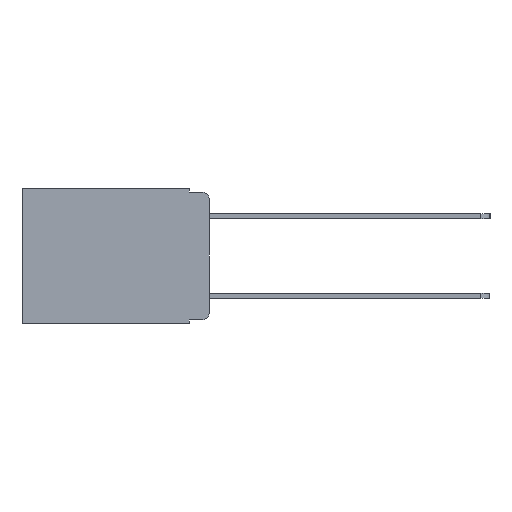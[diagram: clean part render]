
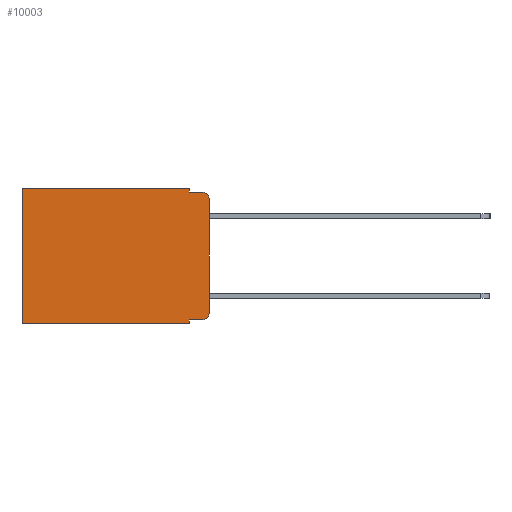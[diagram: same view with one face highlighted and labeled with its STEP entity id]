
A CAD part, left-side view. The second image highlights one B-rep face of the part: STEP entity #10003.
In plain terms, the highlighted planar face has unit normal (-1, 0, 0).
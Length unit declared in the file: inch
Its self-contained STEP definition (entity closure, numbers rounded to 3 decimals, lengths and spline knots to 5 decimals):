
#554 = ORIENTED_EDGE ( 'NONE', *, *, #4159, .T. ) ;
#816 = VERTEX_POINT ( 'NONE', #14394 ) ;
#1519 = VECTOR ( 'NONE', #15844, 39.37008 ) ;
#1655 = CARTESIAN_POINT ( 'NONE',  ( 0.298, 0.051, -0.01 ) ) ;
#2200 = DIRECTION ( 'NONE',  ( 0., 0., -1. ) ) ;
#2256 = EDGE_CURVE ( 'NONE', #7905, #13920, #16544, .T. ) ;
#2439 = LINE ( 'NONE', #9801, #15639 ) ;
#2563 = VERTEX_POINT ( 'NONE', #10602 ) ;
#3009 = CARTESIAN_POINT ( 'NONE',  ( 0.298, 0., -0.343 ) ) ;
#3080 = CARTESIAN_POINT ( 'NONE',  ( 0.298, 0.051, 0. ) ) ;
#3107 = ORIENTED_EDGE ( 'NONE', *, *, #4132, .F. ) ;
#3356 = ORIENTED_EDGE ( 'NONE', *, *, #2256, .T. ) ;
#3357 = CARTESIAN_POINT ( 'NONE',  ( 0.298, 0., -0.313 ) ) ;
#3617 = ORIENTED_EDGE ( 'NONE', *, *, #4163, .F. ) ;
#3933 = EDGE_CURVE ( 'NONE', #5489, #11102, #9654, .T. ) ;
#4132 = EDGE_CURVE ( 'NONE', #12912, #11701, #13716, .T. ) ;
#4159 = EDGE_CURVE ( 'NONE', #12912, #816, #13006, .T. ) ;
#4163 = EDGE_CURVE ( 'NONE', #6048, #816, #2439, .T. ) ;
#4187 = EDGE_CURVE ( 'NONE', #7905, #6048, #15972, .T. ) ;
#4191 = EDGE_CURVE ( 'NONE', #13920, #11102, #12296, .T. ) ;
#4195 = EDGE_CURVE ( 'NONE', #6336, #5489, #14955, .T. ) ;
#4214 = EDGE_CURVE ( 'NONE', #6336, #2563, #8811, .T. ) ;
#4217 = EDGE_CURVE ( 'NONE', #2563, #11701, #11612, .T. ) ;
#4826 = DIRECTION ( 'NONE',  ( 0., 0., -1. ) ) ;
#4884 = CARTESIAN_POINT ( 'NONE',  ( 0.298, 0.051, 0. ) ) ;
#4959 = ORIENTED_EDGE ( 'NONE', *, *, #4217, .T. ) ;
#5005 = VECTOR ( 'NONE', #4826, 39.37008 ) ;
#5280 = ORIENTED_EDGE ( 'NONE', *, *, #4214, .T. ) ;
#5489 = VERTEX_POINT ( 'NONE', #15394 ) ;
#5558 = DIRECTION ( 'NONE',  ( 0., 0., -1. ) ) ;
#5625 = CARTESIAN_POINT ( 'NONE',  ( 0.298, 0., 0. ) ) ;
#5723 = CARTESIAN_POINT ( 'NONE',  ( 0.298, 0., 0. ) ) ;
#5915 = CARTESIAN_POINT ( 'NONE',  ( 0.298, 0., -0.03 ) ) ;
#5949 = ORIENTED_EDGE ( 'NONE', *, *, #3933, .F. ) ;
#6048 = VERTEX_POINT ( 'NONE', #1655 ) ;
#6069 = DIRECTION ( 'NONE',  ( 0., -1., 0. ) ) ;
#6336 = VERTEX_POINT ( 'NONE', #8423 ) ;
#6429 = VECTOR ( 'NONE', #10568, 39.37008 ) ;
#7172 = VECTOR ( 'NONE', #12456, 39.37008 ) ;
#7332 = VECTOR ( 'NONE', #5558, 39.37008 ) ;
#7707 = DIRECTION ( 'NONE',  ( 0., 0., -1. ) ) ;
#7724 = DIRECTION ( 'NONE',  ( -1., 0., 0. ) ) ;
#7732 = CARTESIAN_POINT ( 'NONE',  ( 0.298, 0.02, -0.313 ) ) ;
#7905 = VERTEX_POINT ( 'NONE', #3080 ) ;
#8303 = AXIS2_PLACEMENT_3D ( 'NONE', #9540, #9524, #8873 ) ;
#8423 = CARTESIAN_POINT ( 'NONE',  ( 0.298, 0.051, -0.333 ) ) ;
#8775 = ORIENTED_EDGE ( 'NONE', *, *, #4187, .F. ) ;
#8811 = LINE ( 'NONE', #12923, #14241 ) ;
#8853 = DIRECTION ( 'NONE',  ( 0., -1., 0. ) ) ;
#8873 = DIRECTION ( 'NONE',  ( 0., 0., -1. ) ) ;
#9524 = DIRECTION ( 'NONE',  ( -1., 0., 0. ) ) ;
#9540 = CARTESIAN_POINT ( 'NONE',  ( 0.298, 0.02, -0.03 ) ) ;
#9553 = AXIS2_PLACEMENT_3D ( 'NONE', #5723, #16585, #9894 ) ;
#9654 = LINE ( 'NONE', #3009, #6429 ) ;
#9801 = CARTESIAN_POINT ( 'NONE',  ( 0.298, 0.051, -0.01 ) ) ;
#9894 = DIRECTION ( 'NONE',  ( 0., 0., -1. ) ) ;
#10003 = ADVANCED_FACE ( 'NONE', ( #15255 ), #12108, .F. ) ;
#10078 = EDGE_LOOP ( 'NONE', ( #3107, #554, #3617, #8775, #3356, #12429, #5949, #15469, #5280, #4959 ) ) ;
#10181 = CARTESIAN_POINT ( 'NONE',  ( 0.298, 0., 0. ) ) ;
#10568 = DIRECTION ( 'NONE',  ( 0., 1., 0. ) ) ;
#10602 = CARTESIAN_POINT ( 'NONE',  ( 0.298, 0.02, -0.333 ) ) ;
#11102 = VERTEX_POINT ( 'NONE', #15483 ) ;
#11612 = CIRCLE ( 'NONE', #12303, 0.02 ) ;
#11701 = VERTEX_POINT ( 'NONE', #3357 ) ;
#11951 = VECTOR ( 'NONE', #2200, 39.37008 ) ;
#12108 = PLANE ( 'NONE',  #9553 ) ;
#12296 = LINE ( 'NONE', #14493, #11951 ) ;
#12303 = AXIS2_PLACEMENT_3D ( 'NONE', #7732, #7724, #7707 ) ;
#12429 = ORIENTED_EDGE ( 'NONE', *, *, #4191, .T. ) ;
#12456 = DIRECTION ( 'NONE',  ( 0., 1., 0. ) ) ;
#12912 = VERTEX_POINT ( 'NONE', #5915 ) ;
#12923 = CARTESIAN_POINT ( 'NONE',  ( 0.298, 0.051, -0.333 ) ) ;
#13006 = CIRCLE ( 'NONE', #8303, 0.02 ) ;
#13716 = LINE ( 'NONE', #5625, #7332 ) ;
#13920 = VERTEX_POINT ( 'NONE', #16578 ) ;
#14241 = VECTOR ( 'NONE', #6069, 39.37008 ) ;
#14394 = CARTESIAN_POINT ( 'NONE',  ( 0.298, 0.02, -0.01 ) ) ;
#14493 = CARTESIAN_POINT ( 'NONE',  ( 0.298, 0.473, 0. ) ) ;
#14955 = LINE ( 'NONE', #4884, #5005 ) ;
#15255 = FACE_OUTER_BOUND ( 'NONE', #10078, .T. ) ;
#15394 = CARTESIAN_POINT ( 'NONE',  ( 0.298, 0.051, -0.343 ) ) ;
#15469 = ORIENTED_EDGE ( 'NONE', *, *, #4195, .F. ) ;
#15483 = CARTESIAN_POINT ( 'NONE',  ( 0.298, 0.473, -0.343 ) ) ;
#15639 = VECTOR ( 'NONE', #8853, 39.37008 ) ;
#15844 = DIRECTION ( 'NONE',  ( 0., 0., -1. ) ) ;
#15857 = CARTESIAN_POINT ( 'NONE',  ( 0.298, 0.051, 0. ) ) ;
#15972 = LINE ( 'NONE', #15857, #1519 ) ;
#16544 = LINE ( 'NONE', #10181, #7172 ) ;
#16578 = CARTESIAN_POINT ( 'NONE',  ( 0.298, 0.473, 0. ) ) ;
#16585 = DIRECTION ( 'NONE',  ( 1., 0., 0. ) ) ;
